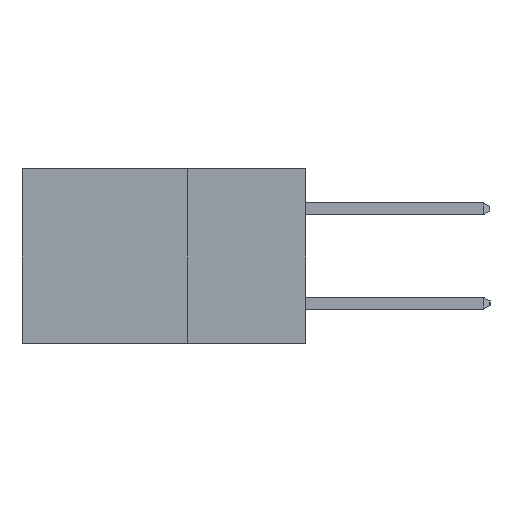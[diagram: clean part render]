
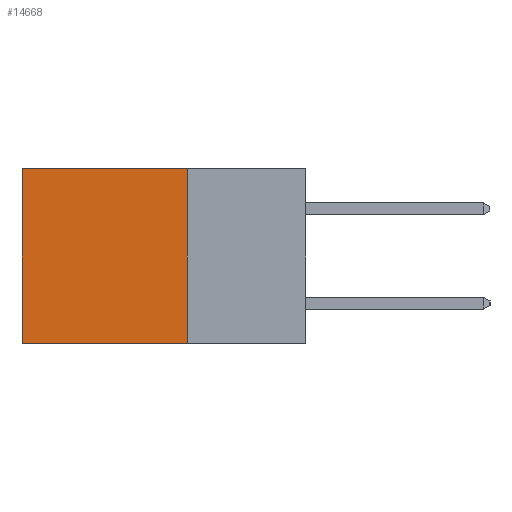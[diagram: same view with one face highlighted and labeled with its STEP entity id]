
A CAD part, left-side view. The second image highlights one B-rep face of the part: STEP entity #14668.
In plain terms, the highlighted planar face has unit normal (-1, 0, 0).
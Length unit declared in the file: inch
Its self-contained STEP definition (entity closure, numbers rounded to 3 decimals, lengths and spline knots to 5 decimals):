
#25 = ORIENTED_EDGE ( 'NONE', *, *, #11820, .F. ) ;
#1626 = DIRECTION ( 'NONE',  ( 0., 1., 0. ) ) ;
#2259 = CARTESIAN_POINT ( 'NONE',  ( 0.2615, 0.6, -0.37 ) ) ;
#3741 = DIRECTION ( 'NONE',  ( 0., 0., -1. ) ) ;
#4501 = CARTESIAN_POINT ( 'NONE',  ( 0.2615, 0.25, -0.37 ) ) ;
#5034 = LINE ( 'NONE', #13320, #10261 ) ;
#5547 = CARTESIAN_POINT ( 'NONE',  ( 0.2615, 0.6, 0. ) ) ;
#5981 = VERTEX_POINT ( 'NONE', #18896 ) ;
#6069 = VECTOR ( 'NONE', #23040, 39.37008 ) ;
#6181 = FACE_OUTER_BOUND ( 'NONE', #22331, .T. ) ;
#6469 = DIRECTION ( 'NONE',  ( 0., 0., -1. ) ) ;
#8109 = DIRECTION ( 'NONE',  ( 0., 0., -1. ) ) ;
#9472 = LINE ( 'NONE', #2259, #10079 ) ;
#10079 = VECTOR ( 'NONE', #8109, 39.37008 ) ;
#10261 = VECTOR ( 'NONE', #1626, 39.37008 ) ;
#11005 = VERTEX_POINT ( 'NONE', #5547 ) ;
#11820 = EDGE_CURVE ( 'NONE', #23285, #23708, #23302, .T. ) ;
#13320 = CARTESIAN_POINT ( 'NONE',  ( 0.2615, 0.25, 0. ) ) ;
#13402 = CARTESIAN_POINT ( 'NONE',  ( 0.2615, 0.25, 0. ) ) ;
#14668 = ADVANCED_FACE ( 'NONE', ( #6181 ), #23818, .F. ) ;
#16549 = CARTESIAN_POINT ( 'NONE',  ( 0.2615, 0.25, -0.37 ) ) ;
#17435 = CARTESIAN_POINT ( 'NONE',  ( 0.2615, 0.25, -0.37 ) ) ;
#17786 = AXIS2_PLACEMENT_3D ( 'NONE', #4501, #18186, #6469 ) ;
#18063 = EDGE_CURVE ( 'NONE', #23708, #5981, #21619, .T. ) ;
#18186 = DIRECTION ( 'NONE',  ( 1., 0., 0. ) ) ;
#18896 = CARTESIAN_POINT ( 'NONE',  ( 0.2615, 0.6, -0.37 ) ) ;
#19361 = ORIENTED_EDGE ( 'NONE', *, *, #24881, .T. ) ;
#20082 = ORIENTED_EDGE ( 'NONE', *, *, #20767, .T. ) ;
#20767 = EDGE_CURVE ( 'NONE', #23285, #11005, #5034, .T. ) ;
#21145 = CARTESIAN_POINT ( 'NONE',  ( 0.2615, 0.25, -0.37 ) ) ;
#21619 = LINE ( 'NONE', #21145, #6069 ) ;
#22331 = EDGE_LOOP ( 'NONE', ( #19361, #24020, #25, #20082 ) ) ;
#22702 = VECTOR ( 'NONE', #3741, 39.37008 ) ;
#23040 = DIRECTION ( 'NONE',  ( 0., 1., 0. ) ) ;
#23285 = VERTEX_POINT ( 'NONE', #13402 ) ;
#23302 = LINE ( 'NONE', #17435, #22702 ) ;
#23708 = VERTEX_POINT ( 'NONE', #16549 ) ;
#23818 = PLANE ( 'NONE',  #17786 ) ;
#24020 = ORIENTED_EDGE ( 'NONE', *, *, #18063, .F. ) ;
#24881 = EDGE_CURVE ( 'NONE', #11005, #5981, #9472, .T. ) ;
